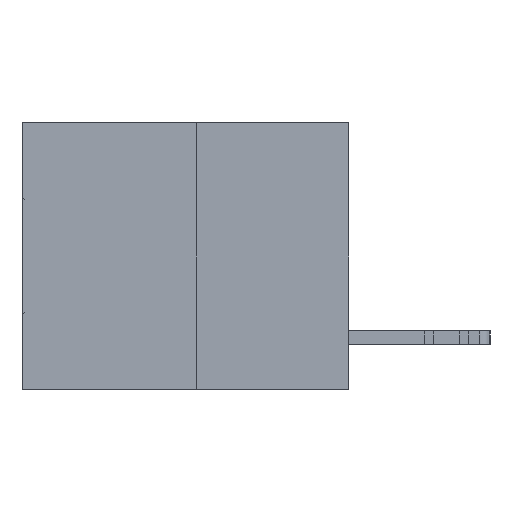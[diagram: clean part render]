
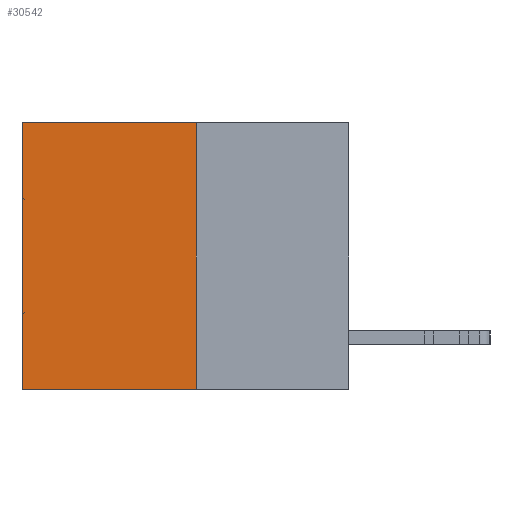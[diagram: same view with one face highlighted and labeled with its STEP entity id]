
A CAD part, left-side view. The second image highlights one B-rep face of the part: STEP entity #30542.
In plain terms, the highlighted planar face has unit normal (-1, 0, 0).
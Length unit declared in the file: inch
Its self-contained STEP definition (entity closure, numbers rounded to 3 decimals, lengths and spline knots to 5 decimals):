
#1663 = EDGE_CURVE ( 'NONE', #23554, #17893, #13610, .T. ) ;
#2808 = ORIENTED_EDGE ( 'NONE', *, *, #29510, .F. ) ;
#3276 = CARTESIAN_POINT ( 'NONE',  ( 0.3165, 0.6, 0. ) ) ;
#3388 = DIRECTION ( 'NONE',  ( 0., 1., 0. ) ) ;
#6375 = DIRECTION ( 'NONE',  ( 0., 0., -1. ) ) ;
#6981 = DIRECTION ( 'NONE',  ( 1., 0., 0. ) ) ;
#7134 = VECTOR ( 'NONE', #32713, 39.37008 ) ;
#7786 = CARTESIAN_POINT ( 'NONE',  ( 0.3165, 0.6, -0.49 ) ) ;
#11167 = FACE_OUTER_BOUND ( 'NONE', #31194, .T. ) ;
#11230 = ORIENTED_EDGE ( 'NONE', *, *, #1663, .T. ) ;
#11511 = CARTESIAN_POINT ( 'NONE',  ( 0.3165, 0.28, -0.49 ) ) ;
#11811 = DIRECTION ( 'NONE',  ( 0., 0., -1. ) ) ;
#12250 = ORIENTED_EDGE ( 'NONE', *, *, #29656, .F. ) ;
#12318 = CARTESIAN_POINT ( 'NONE',  ( 0.3165, 0.28, -0.49 ) ) ;
#12440 = PLANE ( 'NONE',  #27892 ) ;
#13610 = LINE ( 'NONE', #14062, #23888 ) ;
#13866 = CARTESIAN_POINT ( 'NONE',  ( 0.3165, 0.28, -0.49 ) ) ;
#14062 = CARTESIAN_POINT ( 'NONE',  ( 0.3165, 0.6, -0.49 ) ) ;
#15882 = LINE ( 'NONE', #16241, #17462 ) ;
#16241 = CARTESIAN_POINT ( 'NONE',  ( 0.3165, 0.28, 0. ) ) ;
#17269 = LINE ( 'NONE', #12318, #7134 ) ;
#17353 = DIRECTION ( 'NONE',  ( 0., 0., -1. ) ) ;
#17462 = VECTOR ( 'NONE', #3388, 39.37008 ) ;
#17893 = VERTEX_POINT ( 'NONE', #7786 ) ;
#21261 = VERTEX_POINT ( 'NONE', #11511 ) ;
#23554 = VERTEX_POINT ( 'NONE', #3276 ) ;
#23888 = VECTOR ( 'NONE', #11811, 39.37008 ) ;
#25702 = VECTOR ( 'NONE', #6375, 39.37008 ) ;
#26817 = VERTEX_POINT ( 'NONE', #27524 ) ;
#27524 = CARTESIAN_POINT ( 'NONE',  ( 0.3165, 0.28, 0. ) ) ;
#27892 = AXIS2_PLACEMENT_3D ( 'NONE', #30191, #6981, #17353 ) ;
#29510 = EDGE_CURVE ( 'NONE', #21261, #17893, #17269, .T. ) ;
#29656 = EDGE_CURVE ( 'NONE', #26817, #21261, #32484, .T. ) ;
#30191 = CARTESIAN_POINT ( 'NONE',  ( 0.3165, 0.28, -0.49 ) ) ;
#30542 = ADVANCED_FACE ( 'NONE', ( #11167 ), #12440, .F. ) ;
#30761 = ORIENTED_EDGE ( 'NONE', *, *, #31556, .T. ) ;
#31194 = EDGE_LOOP ( 'NONE', ( #11230, #2808, #12250, #30761 ) ) ;
#31556 = EDGE_CURVE ( 'NONE', #26817, #23554, #15882, .T. ) ;
#32484 = LINE ( 'NONE', #13866, #25702 ) ;
#32713 = DIRECTION ( 'NONE',  ( 0., 1., 0. ) ) ;
